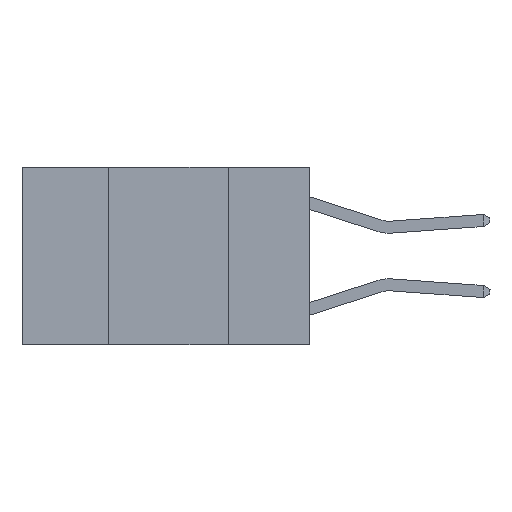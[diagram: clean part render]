
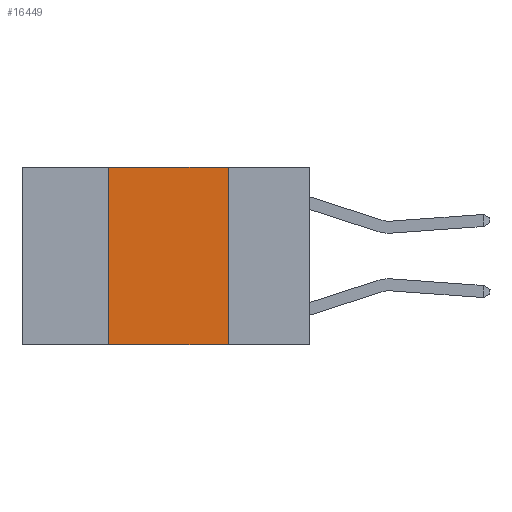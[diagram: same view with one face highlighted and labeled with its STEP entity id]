
A CAD part, left-side view. The second image highlights one B-rep face of the part: STEP entity #16449.
In plain terms, the highlighted planar face has unit normal (-1, 0, 0).
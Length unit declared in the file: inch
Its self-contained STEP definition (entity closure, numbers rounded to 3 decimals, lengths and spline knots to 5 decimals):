
#1074 = LINE ( 'NONE', #1433, #10666 ) ;
#1223 = CARTESIAN_POINT ( 'NONE',  ( 0., 0.42, 0. ) ) ;
#1433 = CARTESIAN_POINT ( 'NONE',  ( 0., 0.6, 0. ) ) ;
#2374 = CARTESIAN_POINT ( 'NONE',  ( 0., 0.6, -0.37 ) ) ;
#3065 = VECTOR ( 'NONE', #10002, 39.37008 ) ;
#4023 = PLANE ( 'NONE',  #6165 ) ;
#5181 = ORIENTED_EDGE ( 'NONE', *, *, #8019, .T. ) ;
#5925 = DIRECTION ( 'NONE',  ( 1., 0., 0. ) ) ;
#6165 = AXIS2_PLACEMENT_3D ( 'NONE', #17323, #5925, #19216 ) ;
#6235 = FACE_OUTER_BOUND ( 'NONE', #17223, .T. ) ;
#7736 = CARTESIAN_POINT ( 'NONE',  ( 0., 0.17, -0.37 ) ) ;
#8019 = EDGE_CURVE ( 'NONE', #22982, #14656, #9513, .T. ) ;
#8284 = DIRECTION ( 'NONE',  ( 0., 0., 1. ) ) ;
#8381 = EDGE_CURVE ( 'NONE', #9492, #23611, #1074, .T. ) ;
#8419 = CARTESIAN_POINT ( 'NONE',  ( 0., 0.42, -0.37 ) ) ;
#8449 = ORIENTED_EDGE ( 'NONE', *, *, #16610, .F. ) ;
#9371 = LINE ( 'NONE', #17558, #3065 ) ;
#9492 = VERTEX_POINT ( 'NONE', #1223 ) ;
#9513 = LINE ( 'NONE', #2374, #12809 ) ;
#10002 = DIRECTION ( 'NONE',  ( 0., 0., -1. ) ) ;
#10666 = VECTOR ( 'NONE', #18611, 39.37008 ) ;
#11724 = ORIENTED_EDGE ( 'NONE', *, *, #20333, .F. ) ;
#12225 = LINE ( 'NONE', #19618, #21007 ) ;
#12809 = VECTOR ( 'NONE', #23251, 39.37008 ) ;
#14656 = VERTEX_POINT ( 'NONE', #7736 ) ;
#16449 = ADVANCED_FACE ( 'NONE', ( #6235 ), #4023, .F. ) ;
#16610 = EDGE_CURVE ( 'NONE', #22982, #9492, #12225, .T. ) ;
#17223 = EDGE_LOOP ( 'NONE', ( #11724, #23485, #8449, #5181 ) ) ;
#17323 = CARTESIAN_POINT ( 'NONE',  ( 0., 0.6, 0. ) ) ;
#17558 = CARTESIAN_POINT ( 'NONE',  ( 0., 0.17, 0. ) ) ;
#18611 = DIRECTION ( 'NONE',  ( 0., -1., 0. ) ) ;
#19216 = DIRECTION ( 'NONE',  ( 0., 0., -1. ) ) ;
#19618 = CARTESIAN_POINT ( 'NONE',  ( 0., 0.42, 0. ) ) ;
#20333 = EDGE_CURVE ( 'NONE', #23611, #14656, #9371, .T. ) ;
#21007 = VECTOR ( 'NONE', #8284, 39.37008 ) ;
#22982 = VERTEX_POINT ( 'NONE', #8419 ) ;
#23209 = CARTESIAN_POINT ( 'NONE',  ( 0., 0.17, 0. ) ) ;
#23251 = DIRECTION ( 'NONE',  ( 0., -1., 0. ) ) ;
#23485 = ORIENTED_EDGE ( 'NONE', *, *, #8381, .F. ) ;
#23611 = VERTEX_POINT ( 'NONE', #23209 ) ;
